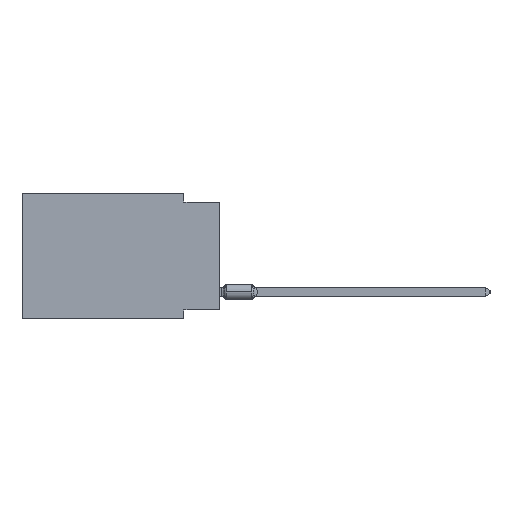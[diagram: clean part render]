
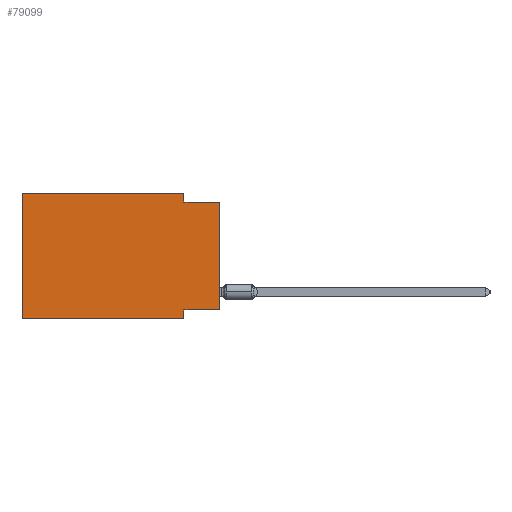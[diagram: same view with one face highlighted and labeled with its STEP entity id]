
A CAD part, left-side view. The second image highlights one B-rep face of the part: STEP entity #79099.
In plain terms, the highlighted planar face has unit normal (-1, 0, 0).
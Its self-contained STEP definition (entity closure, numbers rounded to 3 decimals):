
#3613 = LINE ( 'NONE', #37119, #59101 ) ;
#4860 = DIRECTION ( 'NONE',  ( 0., 0., -1. ) ) ;
#5506 = CARTESIAN_POINT ( 'NONE',  ( 0., 13.97, 0. ) ) ;
#8086 = VECTOR ( 'NONE', #44463, 1000. ) ;
#10944 = LINE ( 'NONE', #104339, #8086 ) ;
#11325 = VERTEX_POINT ( 'NONE', #63739 ) ;
#17748 = ORIENTED_EDGE ( 'NONE', *, *, #55136, .F. ) ;
#18202 = EDGE_CURVE ( 'NONE', #68192, #107876, #37062, .T. ) ;
#22106 = LINE ( 'NONE', #96303, #37525 ) ;
#22360 = VECTOR ( 'NONE', #61346, 1000. ) ;
#27153 = VECTOR ( 'NONE', #4860, 1000. ) ;
#28996 = CARTESIAN_POINT ( 'NONE',  ( 0., 2.54, 0. ) ) ;
#32662 = EDGE_CURVE ( 'NONE', #101449, #11325, #81219, .T. ) ;
#33804 = CARTESIAN_POINT ( 'NONE',  ( 0., 2.54, -8.89 ) ) ;
#37062 = LINE ( 'NONE', #53562, #70485 ) ;
#37119 = CARTESIAN_POINT ( 'NONE',  ( 0., 0., -8.255 ) ) ;
#37525 = VECTOR ( 'NONE', #64418, 1000. ) ;
#40473 = LINE ( 'NONE', #56424, #63134 ) ;
#42721 = VERTEX_POINT ( 'NONE', #89514 ) ;
#44463 = DIRECTION ( 'NONE',  ( 0., 0., 1. ) ) ;
#47423 = EDGE_CURVE ( 'NONE', #87479, #107876, #40473, .T. ) ;
#48885 = DIRECTION ( 'NONE',  ( 0., 0., -1. ) ) ;
#50095 = CARTESIAN_POINT ( 'NONE',  ( 0., 2.54, -8.255 ) ) ;
#52503 = ORIENTED_EDGE ( 'NONE', *, *, #47423, .F. ) ;
#53562 = CARTESIAN_POINT ( 'NONE',  ( 0., 13.97, -8.89 ) ) ;
#55136 = EDGE_CURVE ( 'NONE', #68192, #76058, #10944, .T. ) ;
#55486 = CARTESIAN_POINT ( 'NONE',  ( 0., 0., -8.255 ) ) ;
#56424 = CARTESIAN_POINT ( 'NONE',  ( 0., 2.54, -8.89 ) ) ;
#57137 = LINE ( 'NONE', #106624, #62807 ) ;
#59101 = VECTOR ( 'NONE', #70657, 1000. ) ;
#61346 = DIRECTION ( 'NONE',  ( 0., -1., 0. ) ) ;
#62807 = VECTOR ( 'NONE', #81337, 1000. ) ;
#63134 = VECTOR ( 'NONE', #65227, 1000. ) ;
#63739 = CARTESIAN_POINT ( 'NONE',  ( 0., 2.54, -0.635 ) ) ;
#64418 = DIRECTION ( 'NONE',  ( 0., 0., 1. ) ) ;
#64497 = ORIENTED_EDGE ( 'NONE', *, *, #76715, .F. ) ;
#65227 = DIRECTION ( 'NONE',  ( 0., 0., -1. ) ) ;
#65388 = PLANE ( 'NONE',  #90244 ) ;
#68192 = VERTEX_POINT ( 'NONE', #90126 ) ;
#68805 = ORIENTED_EDGE ( 'NONE', *, *, #32662, .F. ) ;
#69591 = CARTESIAN_POINT ( 'NONE',  ( 0., 0., -0.635 ) ) ;
#70485 = VECTOR ( 'NONE', #94794, 1000. ) ;
#70640 = ORIENTED_EDGE ( 'NONE', *, *, #70902, .F. ) ;
#70657 = DIRECTION ( 'NONE',  ( 0., 1., 0. ) ) ;
#70662 = LINE ( 'NONE', #69591, #22360 ) ;
#70902 = EDGE_CURVE ( 'NONE', #76058, #101449, #57137, .T. ) ;
#73968 = EDGE_LOOP ( 'NONE', ( #74601, #64497, #68805, #70640, #17748, #99777, #52503, #94799 ) ) ;
#74601 = ORIENTED_EDGE ( 'NONE', *, *, #95396, .T. ) ;
#76058 = VERTEX_POINT ( 'NONE', #104870 ) ;
#76715 = EDGE_CURVE ( 'NONE', #11325, #42721, #70662, .T. ) ;
#79099 = ADVANCED_FACE ( 'NONE', ( #97824 ), #65388, .F. ) ;
#81219 = LINE ( 'NONE', #89466, #27153 ) ;
#81337 = DIRECTION ( 'NONE',  ( 0., -1., 0. ) ) ;
#87479 = VERTEX_POINT ( 'NONE', #50095 ) ;
#89466 = CARTESIAN_POINT ( 'NONE',  ( 0., 2.54, 0. ) ) ;
#89514 = CARTESIAN_POINT ( 'NONE',  ( 0., 0., -0.635 ) ) ;
#90111 = DIRECTION ( 'NONE',  ( 1., 0., 0. ) ) ;
#90126 = CARTESIAN_POINT ( 'NONE',  ( 0., 13.97, -8.89 ) ) ;
#90244 = AXIS2_PLACEMENT_3D ( 'NONE', #5506, #90111, #48885 ) ;
#93043 = VERTEX_POINT ( 'NONE', #55486 ) ;
#93778 = EDGE_CURVE ( 'NONE', #93043, #87479, #3613, .T. ) ;
#94794 = DIRECTION ( 'NONE',  ( 0., -1., 0. ) ) ;
#94799 = ORIENTED_EDGE ( 'NONE', *, *, #93778, .F. ) ;
#95396 = EDGE_CURVE ( 'NONE', #93043, #42721, #22106, .T. ) ;
#96303 = CARTESIAN_POINT ( 'NONE',  ( 0., 0., 0. ) ) ;
#97824 = FACE_OUTER_BOUND ( 'NONE', #73968, .T. ) ;
#99777 = ORIENTED_EDGE ( 'NONE', *, *, #18202, .T. ) ;
#101449 = VERTEX_POINT ( 'NONE', #28996 ) ;
#104339 = CARTESIAN_POINT ( 'NONE',  ( 0., 13.97, 0. ) ) ;
#104870 = CARTESIAN_POINT ( 'NONE',  ( 0., 13.97, 0. ) ) ;
#106624 = CARTESIAN_POINT ( 'NONE',  ( 0., 13.97, 0. ) ) ;
#107876 = VERTEX_POINT ( 'NONE', #33804 ) ;
